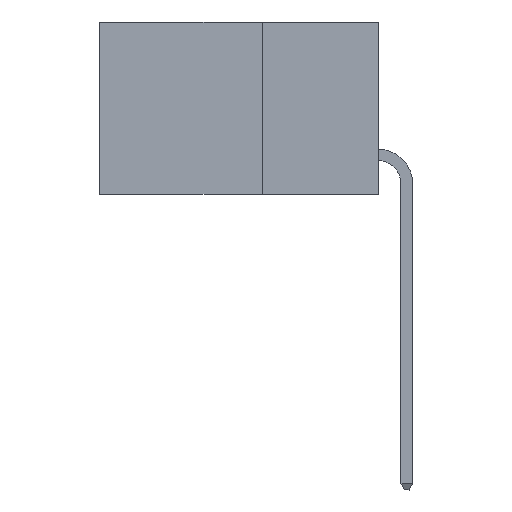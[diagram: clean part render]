
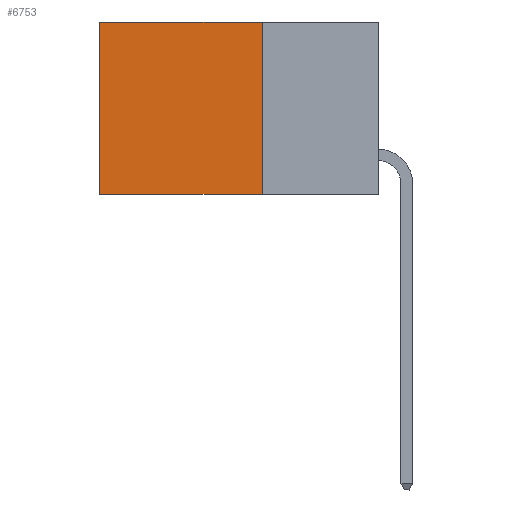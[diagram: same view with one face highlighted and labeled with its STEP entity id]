
A CAD part, left-side view. The second image highlights one B-rep face of the part: STEP entity #6753.
In plain terms, the highlighted planar face has unit normal (-1, 0, 0).
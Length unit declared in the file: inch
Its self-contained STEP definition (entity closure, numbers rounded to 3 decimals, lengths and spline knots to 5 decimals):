
#98 = CARTESIAN_POINT ( 'NONE',  ( 0.298, 0.25, 0. ) ) ;
#541 = EDGE_CURVE ( 'NONE', #857, #3031, #9366, .T. ) ;
#689 = DIRECTION ( 'NONE',  ( 0., 0., -1. ) ) ;
#721 = ORIENTED_EDGE ( 'NONE', *, *, #11458, .T. ) ;
#857 = VERTEX_POINT ( 'NONE', #98 ) ;
#1089 = VERTEX_POINT ( 'NONE', #8373 ) ;
#1610 = AXIS2_PLACEMENT_3D ( 'NONE', #11286, #11344, #3185 ) ;
#1762 = PLANE ( 'NONE',  #1610 ) ;
#2388 = VECTOR ( 'NONE', #5094, 39.37008 ) ;
#3031 = VERTEX_POINT ( 'NONE', #7943 ) ;
#3185 = DIRECTION ( 'NONE',  ( 0., 0., -1. ) ) ;
#4281 = ORIENTED_EDGE ( 'NONE', *, *, #7595, .F. ) ;
#4422 = VERTEX_POINT ( 'NONE', #17067 ) ;
#4706 = LINE ( 'NONE', #10658, #11905 ) ;
#5081 = VECTOR ( 'NONE', #11529, 39.37008 ) ;
#5094 = DIRECTION ( 'NONE',  ( 0., 1., 0. ) ) ;
#6753 = ADVANCED_FACE ( 'NONE', ( #7772 ), #1762, .F. ) ;
#7586 = ORIENTED_EDGE ( 'NONE', *, *, #12666, .T. ) ;
#7595 = EDGE_CURVE ( 'NONE', #3031, #1089, #13184, .T. ) ;
#7772 = FACE_OUTER_BOUND ( 'NONE', #9233, .T. ) ;
#7943 = CARTESIAN_POINT ( 'NONE',  ( 0.298, 0.25, -0.37 ) ) ;
#8373 = CARTESIAN_POINT ( 'NONE',  ( 0.298, 0.6, -0.37 ) ) ;
#8741 = LINE ( 'NONE', #16486, #5081 ) ;
#9233 = EDGE_LOOP ( 'NONE', ( #721, #4281, #9734, #7586 ) ) ;
#9366 = LINE ( 'NONE', #14412, #12064 ) ;
#9734 = ORIENTED_EDGE ( 'NONE', *, *, #541, .F. ) ;
#10658 = CARTESIAN_POINT ( 'NONE',  ( 0.298, 0.6, 0. ) ) ;
#11286 = CARTESIAN_POINT ( 'NONE',  ( 0.298, 0.25, 0. ) ) ;
#11344 = DIRECTION ( 'NONE',  ( 1., 0., 0. ) ) ;
#11458 = EDGE_CURVE ( 'NONE', #4422, #1089, #4706, .T. ) ;
#11529 = DIRECTION ( 'NONE',  ( 0., 1., 0. ) ) ;
#11905 = VECTOR ( 'NONE', #11979, 39.37008 ) ;
#11979 = DIRECTION ( 'NONE',  ( 0., 0., -1. ) ) ;
#12064 = VECTOR ( 'NONE', #689, 39.37008 ) ;
#12666 = EDGE_CURVE ( 'NONE', #857, #4422, #8741, .T. ) ;
#13184 = LINE ( 'NONE', #14383, #2388 ) ;
#14383 = CARTESIAN_POINT ( 'NONE',  ( 0.298, 0.25, -0.37 ) ) ;
#14412 = CARTESIAN_POINT ( 'NONE',  ( 0.298, 0.25, 0. ) ) ;
#16486 = CARTESIAN_POINT ( 'NONE',  ( 0.298, 0.25, 0. ) ) ;
#17067 = CARTESIAN_POINT ( 'NONE',  ( 0.298, 0.6, 0. ) ) ;
